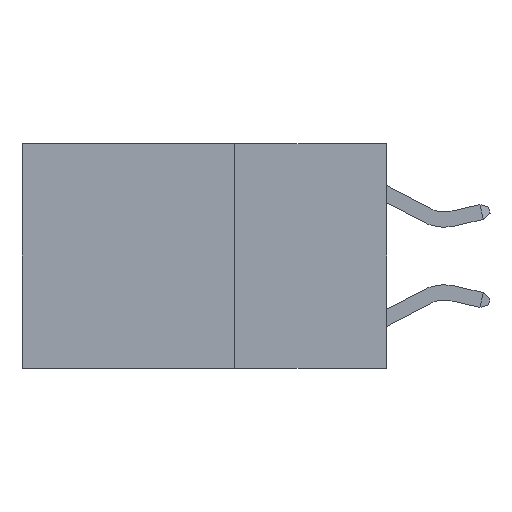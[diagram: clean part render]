
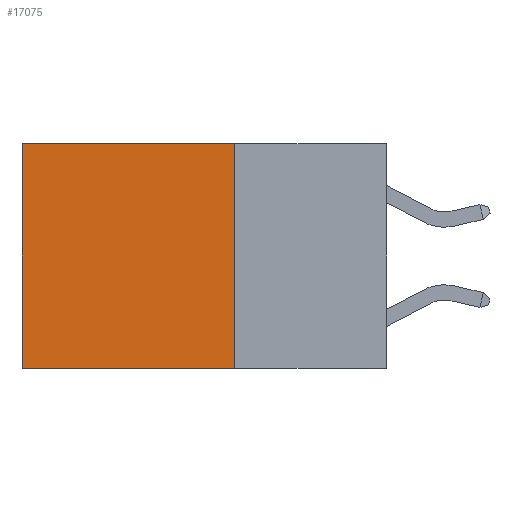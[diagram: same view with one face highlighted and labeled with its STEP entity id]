
A CAD part, left-side view. The second image highlights one B-rep face of the part: STEP entity #17075.
In plain terms, the highlighted planar face has unit normal (-1, 0, 0).
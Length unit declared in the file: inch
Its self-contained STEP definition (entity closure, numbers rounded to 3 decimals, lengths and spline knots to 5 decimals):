
#449 = CARTESIAN_POINT ( 'NONE',  ( 0.2625, 0.6, -0.37 ) ) ;
#537 = EDGE_CURVE ( 'NONE', #14627, #8043, #8455, .T. ) ;
#1702 = ORIENTED_EDGE ( 'NONE', *, *, #537, .F. ) ;
#3292 = EDGE_CURVE ( 'NONE', #17938, #14627, #11645, .T. ) ;
#3374 = CARTESIAN_POINT ( 'NONE',  ( 0.2625, 0.25, -0.37 ) ) ;
#3768 = VECTOR ( 'NONE', #9899, 39.37008 ) ;
#3952 = DIRECTION ( 'NONE',  ( 0., 0., -1. ) ) ;
#4899 = EDGE_CURVE ( 'NONE', #10176, #8043, #21411, .T. ) ;
#5616 = DIRECTION ( 'NONE',  ( 0., 0., -1. ) ) ;
#5884 = PLANE ( 'NONE',  #8900 ) ;
#6572 = CARTESIAN_POINT ( 'NONE',  ( 0.2625, 0.25, 0. ) ) ;
#7443 = CARTESIAN_POINT ( 'NONE',  ( 0.2625, 0.25, 0. ) ) ;
#7635 = VECTOR ( 'NONE', #13095, 39.37008 ) ;
#7878 = DIRECTION ( 'NONE',  ( 1., 0., 0. ) ) ;
#8043 = VERTEX_POINT ( 'NONE', #449 ) ;
#8206 = CARTESIAN_POINT ( 'NONE',  ( 0.2625, 0.25, 0. ) ) ;
#8455 = LINE ( 'NONE', #16289, #7635 ) ;
#8900 = AXIS2_PLACEMENT_3D ( 'NONE', #19578, #7878, #13670 ) ;
#9070 = ORIENTED_EDGE ( 'NONE', *, *, #3292, .F. ) ;
#9899 = DIRECTION ( 'NONE',  ( 0., 1., 0. ) ) ;
#10176 = VERTEX_POINT ( 'NONE', #16130 ) ;
#10258 = EDGE_LOOP ( 'NONE', ( #14335, #1702, #9070, #19854 ) ) ;
#11590 = VECTOR ( 'NONE', #5616, 39.37008 ) ;
#11645 = LINE ( 'NONE', #7443, #15784 ) ;
#13095 = DIRECTION ( 'NONE',  ( 0., 1., 0. ) ) ;
#13670 = DIRECTION ( 'NONE',  ( 0., 0., -1. ) ) ;
#14335 = ORIENTED_EDGE ( 'NONE', *, *, #4899, .T. ) ;
#14559 = EDGE_CURVE ( 'NONE', #17938, #10176, #16998, .T. ) ;
#14627 = VERTEX_POINT ( 'NONE', #3374 ) ;
#15784 = VECTOR ( 'NONE', #3952, 39.37008 ) ;
#16130 = CARTESIAN_POINT ( 'NONE',  ( 0.2625, 0.6, 0. ) ) ;
#16289 = CARTESIAN_POINT ( 'NONE',  ( 0.2625, 0.25, -0.37 ) ) ;
#16998 = LINE ( 'NONE', #6572, #3768 ) ;
#17022 = FACE_OUTER_BOUND ( 'NONE', #10258, .T. ) ;
#17075 = ADVANCED_FACE ( 'NONE', ( #17022 ), #5884, .F. ) ;
#17938 = VERTEX_POINT ( 'NONE', #8206 ) ;
#19578 = CARTESIAN_POINT ( 'NONE',  ( 0.2625, 0.25, 0. ) ) ;
#19854 = ORIENTED_EDGE ( 'NONE', *, *, #14559, .T. ) ;
#20304 = CARTESIAN_POINT ( 'NONE',  ( 0.2625, 0.6, 0. ) ) ;
#21411 = LINE ( 'NONE', #20304, #11590 ) ;
